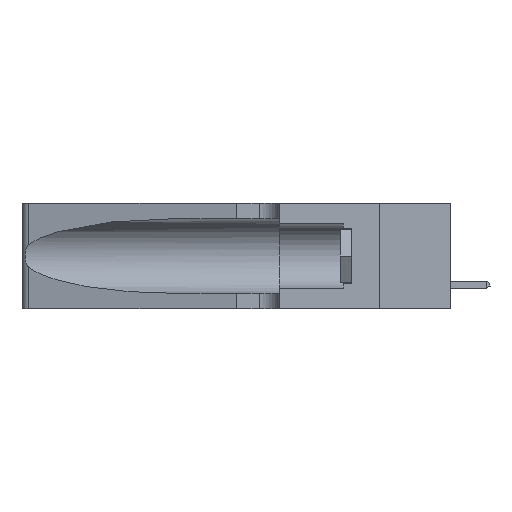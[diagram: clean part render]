
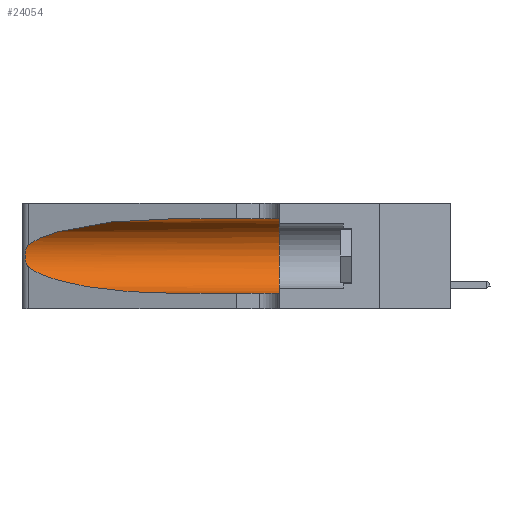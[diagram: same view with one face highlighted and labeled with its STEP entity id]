
A CAD part, left-side view. The second image highlights one B-rep face of the part: STEP entity #24054.
In plain terms, the highlighted cylindrical face has radius 3.308 mm (diameter 6.617 mm), a partial arc.
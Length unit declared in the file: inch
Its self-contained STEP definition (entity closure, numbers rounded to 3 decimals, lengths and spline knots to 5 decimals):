
#234 = CARTESIAN_POINT ( 'NONE',  ( 0.25487, 1.22718, 0.14631 ) ) ;
#638 = EDGE_LOOP ( 'NONE', ( #22006, #25636, #14974, #22471, #8365, #7764 ) ) ;
#1245 = CARTESIAN_POINT ( 'NONE',  ( 0.25639, 1.23184, 0.21858 ) ) ;
#1257 = EDGE_CURVE ( 'NONE', #14561, #18678, #22306, .T. ) ;
#1433 = CARTESIAN_POINT ( 'NONE',  ( 0.26075, 1.23896, 0.19203 ) ) ;
#1671 = CARTESIAN_POINT ( 'NONE',  ( 0.25487, 1.22718, 0.14631 ) ) ;
#2345 = CARTESIAN_POINT ( 'NONE',  ( 0.25487, 1.22718, 0.22369 ) ) ;
#3615 = CARTESIAN_POINT ( 'NONE',  ( 0.1305, 0.72297, 0.05475 ) ) ;
#4304 = VERTEX_POINT ( 'NONE', #25194 ) ;
#4561 = CARTESIAN_POINT ( 'NONE',  ( 0.1305, 0.72297, 0.31525 ) ) ;
#5327 = CARTESIAN_POINT ( 'NONE',  ( 0.25487, 1.22718, 0.22369 ) ) ;
#5487 = DIRECTION ( 'NONE',  ( 0., 0., 1. ) ) ;
#5500 = CARTESIAN_POINT ( 'NONE',  ( 0.25787, 1.23484, 0.2124 ) ) ;
#5647 = EDGE_CURVE ( 'NONE', #20241, #4304, #12408, .T. ) ;
#5771 = EDGE_CURVE ( 'NONE', #20241, #14561, #12371, .T. ) ;
#7090 = AXIS2_PLACEMENT_3D ( 'NONE', #13985, #7729, #5487 ) ;
#7517 = CARTESIAN_POINT ( 'NONE',  ( 0.1305, 0.72297, 0.31525 ) ) ;
#7729 = DIRECTION ( 'NONE',  ( 0., 1., 0. ) ) ;
#7764 = ORIENTED_EDGE ( 'NONE', *, *, #5647, .F. ) ;
#7882 = CARTESIAN_POINT ( 'NONE',  ( 0.2373, 1.15595, 0.08982 ) ) ;
#8049 = VECTOR ( 'NONE', #20820, 39.37008 ) ;
#8365 = ORIENTED_EDGE ( 'NONE', *, *, #27044, .F. ) ;
#8745 = CARTESIAN_POINT ( 'NONE',  ( 0.18966, 0.96281, 0.31525 ) ) ;
#9776 = DIRECTION ( 'NONE',  ( 0., 0., -1. ) ) ;
#10375 = CARTESIAN_POINT ( 'NONE',  ( 0.25487, 1.22718, 0.14631 ) ) ;
#11724 = EDGE_CURVE ( 'NONE', #19197, #23213, #23612, .T. ) ;
#11821 = CARTESIAN_POINT ( 'NONE',  ( 0.1305, 1.61858, 0.05475 ) ) ;
#11974 = CARTESIAN_POINT ( 'NONE',  ( 0.25854, 1.2359, 0.20912 ) ) ;
#12165 = CARTESIAN_POINT ( 'NONE',  ( 0.25856, 1.23593, 0.16098 ) ) ;
#12371 =( BOUNDED_CURVE ( )  B_SPLINE_CURVE ( 3, ( #4561, #8745, #16951, #2345 ),
 .UNSPECIFIED., .F., .T. ) 
 B_SPLINE_CURVE_WITH_KNOTS ( ( 4, 4 ),
 ( 1.5708, 2.84003 ),
 .UNSPECIFIED. ) 
 CURVE ( )  GEOMETRIC_REPRESENTATION_ITEM ( )  RATIONAL_B_SPLINE_CURVE ( ( 1., 0.87, 0.87, 1. ) ) 
 REPRESENTATION_ITEM ( '' )  );
#12408 = LINE ( 'NONE', #18841, #8049 ) ;
#13985 = CARTESIAN_POINT ( 'NONE',  ( 0.1305, 0.35, 0.185 ) ) ;
#14183 = CARTESIAN_POINT ( 'NONE',  ( 0.26017, 1.23833, 0.17102 ) ) ;
#14474 = CARTESIAN_POINT ( 'NONE',  ( 0.26075, 1.23896, 0.178 ) ) ;
#14561 = VERTEX_POINT ( 'NONE', #23348 ) ;
#14974 = ORIENTED_EDGE ( 'NONE', *, *, #24519, .T. ) ;
#15532 = CIRCLE ( 'NONE', #7090, 0.13025 ) ;
#15898 = VECTOR ( 'NONE', #20054, 39.37008 ) ;
#16310 = AXIS2_PLACEMENT_3D ( 'NONE', #24832, #27069, #9776 ) ;
#16951 = CARTESIAN_POINT ( 'NONE',  ( 0.2373, 1.15595, 0.28018 ) ) ;
#18309 =( BOUNDED_CURVE ( )  B_SPLINE_CURVE ( 3, ( #1671, #7882, #22845, #3615 ),
 .UNSPECIFIED., .F., .T. ) 
 B_SPLINE_CURVE_WITH_KNOTS ( ( 4, 4 ),
 ( 3.44316, 4.71239 ),
 .UNSPECIFIED. ) 
 CURVE ( )  GEOMETRIC_REPRESENTATION_ITEM ( )  RATIONAL_B_SPLINE_CURVE ( ( 1., 0.87, 0.87, 1. ) ) 
 REPRESENTATION_ITEM ( '' )  );
#18678 = VERTEX_POINT ( 'NONE', #234 ) ;
#18841 = CARTESIAN_POINT ( 'NONE',  ( 0.1305, 1.61858, 0.31525 ) ) ;
#19197 = VERTEX_POINT ( 'NONE', #25942 ) ;
#20054 = DIRECTION ( 'NONE',  ( 0., -1., 0. ) ) ;
#20241 = VERTEX_POINT ( 'NONE', #7517 ) ;
#20554 = CARTESIAN_POINT ( 'NONE',  ( 0.26018, 1.23835, 0.19895 ) ) ;
#20820 = DIRECTION ( 'NONE',  ( 0., -1., 0. ) ) ;
#20950 = CARTESIAN_POINT ( 'NONE',  ( 0.25555, 1.22993, 0.14849 ) ) ;
#21044 = CARTESIAN_POINT ( 'NONE',  ( 0.25789, 1.23486, 0.15765 ) ) ;
#21102 = FACE_OUTER_BOUND ( 'NONE', #638, .T. ) ;
#21788 = CYLINDRICAL_SURFACE ( 'NONE', #16310, 0.13025 ) ;
#22006 = ORIENTED_EDGE ( 'NONE', *, *, #5771, .T. ) ;
#22306 = B_SPLINE_CURVE_WITH_KNOTS ( 'NONE', 3,
 ( #5327, #26984, #1245, #5500, #11974, #20554, #1433, #14474, #14183, #12165, #21044, #23180, #20950, #10375 ),
 .UNSPECIFIED., .F., .F.,
 ( 4, 2, 2, 2, 2, 2, 4 ),
 ( 0., 0.00027, 0.00053, 0.00107, 0.0016, 0.00187, 0.00214 ),
 .UNSPECIFIED. ) ;
#22471 = ORIENTED_EDGE ( 'NONE', *, *, #11724, .T. ) ;
#22845 = CARTESIAN_POINT ( 'NONE',  ( 0.18966, 0.96281, 0.05475 ) ) ;
#23180 = CARTESIAN_POINT ( 'NONE',  ( 0.25639, 1.23186, 0.15144 ) ) ;
#23213 = VERTEX_POINT ( 'NONE', #25503 ) ;
#23348 = CARTESIAN_POINT ( 'NONE',  ( 0.25487, 1.22718, 0.22369 ) ) ;
#23612 = LINE ( 'NONE', #11821, #15898 ) ;
#24054 = ADVANCED_FACE ( 'NONE', ( #21102 ), #21788, .F. ) ;
#24519 = EDGE_CURVE ( 'NONE', #18678, #19197, #18309, .T. ) ;
#24832 = CARTESIAN_POINT ( 'NONE',  ( 0.1305, 1.61858, 0.185 ) ) ;
#25194 = CARTESIAN_POINT ( 'NONE',  ( 0.1305, 0.35, 0.31525 ) ) ;
#25503 = CARTESIAN_POINT ( 'NONE',  ( 0.1305, 0.35, 0.05475 ) ) ;
#25636 = ORIENTED_EDGE ( 'NONE', *, *, #1257, .T. ) ;
#25942 = CARTESIAN_POINT ( 'NONE',  ( 0.1305, 0.72297, 0.05475 ) ) ;
#26984 = CARTESIAN_POINT ( 'NONE',  ( 0.25555, 1.22994, 0.2215 ) ) ;
#27044 = EDGE_CURVE ( 'NONE', #4304, #23213, #15532, .T. ) ;
#27069 = DIRECTION ( 'NONE',  ( 0., -1., 0. ) ) ;
